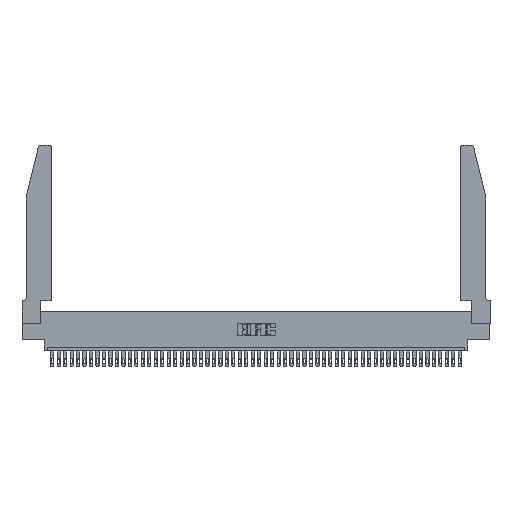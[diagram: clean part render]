
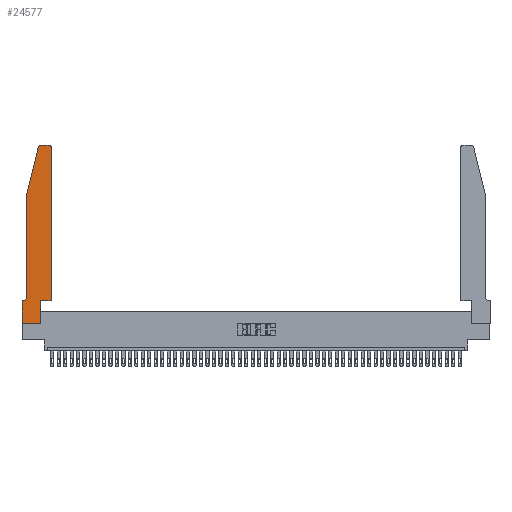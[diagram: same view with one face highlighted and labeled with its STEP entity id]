
A CAD part, top view. The second image highlights one B-rep face of the part: STEP entity #24577.
In plain terms, the highlighted planar face has unit normal (0, 0, 1).
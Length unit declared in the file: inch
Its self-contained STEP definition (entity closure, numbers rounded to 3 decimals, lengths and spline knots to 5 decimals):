
#942 = VERTEX_POINT ( 'NONE', #19809 ) ;
#1291 = VERTEX_POINT ( 'NONE', #23244 ) ;
#3203 = DIRECTION ( 'NONE',  ( 0., 1., 0. ) ) ;
#3223 = EDGE_CURVE ( 'NONE', #942, #12662, #13608, .T. ) ;
#3799 = CARTESIAN_POINT ( 'NONE',  ( 0., 0., 0.37 ) ) ;
#3910 = AXIS2_PLACEMENT_3D ( 'NONE', #31079, #4347, #4511 ) ;
#3929 = DIRECTION ( 'NONE',  ( 0., -1., 0. ) ) ;
#4347 = DIRECTION ( 'NONE',  ( 0., 0., -1. ) ) ;
#4511 = DIRECTION ( 'NONE',  ( -1., 0., 0. ) ) ;
#5018 = CARTESIAN_POINT ( 'NONE',  ( 0.4505, 0.35, 0.37 ) ) ;
#6240 = LINE ( 'NONE', #36328, #31482 ) ;
#6259 = ORIENTED_EDGE ( 'NONE', *, *, #28620, .T. ) ;
#6885 = VERTEX_POINT ( 'NONE', #7023 ) ;
#7023 = CARTESIAN_POINT ( 'NONE',  ( 0.0055, 0.35, 0.37 ) ) ;
#7160 = CARTESIAN_POINT ( 'NONE',  ( 0.2865, 0.35, 0.37 ) ) ;
#7862 = DIRECTION ( 'NONE',  ( 1., 0., 0. ) ) ;
#10143 = CARTESIAN_POINT ( 'NONE',  ( 0.2865, 0.35, 0.37 ) ) ;
#12261 = AXIS2_PLACEMENT_3D ( 'NONE', #22933, #26676, #34442 ) ;
#12622 = EDGE_CURVE ( 'NONE', #23413, #44478, #47587, .T. ) ;
#12662 = VERTEX_POINT ( 'NONE', #14508 ) ;
#13608 = CIRCLE ( 'NONE', #12261, 0.03 ) ;
#14015 = ORIENTED_EDGE ( 'NONE', *, *, #22513, .T. ) ;
#14288 = VERTEX_POINT ( 'NONE', #45154 ) ;
#14508 = CARTESIAN_POINT ( 'NONE',  ( 0.4205, 2.75, 0.37 ) ) ;
#14638 = EDGE_CURVE ( 'NONE', #30166, #6885, #20858, .T. ) ;
#15794 = CARTESIAN_POINT ( 'NONE',  ( 0.0755, 2., 0.37 ) ) ;
#15979 = EDGE_CURVE ( 'NONE', #1291, #19181, #23144, .T. ) ;
#16408 = LINE ( 'NONE', #47495, #32178 ) ;
#16878 = DIRECTION ( 'NONE',  ( -1., 0., 0. ) ) ;
#17016 = ORIENTED_EDGE ( 'NONE', *, *, #12622, .T. ) ;
#17214 = PLANE ( 'NONE',  #42375 ) ;
#17215 = ORIENTED_EDGE ( 'NONE', *, *, #38864, .T. ) ;
#18918 = VECTOR ( 'NONE', #7862, 39.37008 ) ;
#18948 = ORIENTED_EDGE ( 'NONE', *, *, #25670, .T. ) ;
#19085 = AXIS2_PLACEMENT_3D ( 'NONE', #39954, #24548, #27958 ) ;
#19181 = VERTEX_POINT ( 'NONE', #7160 ) ;
#19466 = LINE ( 'NONE', #3799, #18918 ) ;
#19809 = CARTESIAN_POINT ( 'NONE',  ( 0.4505, 2.72, 0.37 ) ) ;
#20485 = LINE ( 'NONE', #33072, #39870 ) ;
#20858 = CIRCLE ( 'NONE', #3910, 0.07 ) ;
#22232 = ORIENTED_EDGE ( 'NONE', *, *, #32112, .T. ) ;
#22513 = EDGE_CURVE ( 'NONE', #43325, #30166, #25351, .T. ) ;
#22933 = CARTESIAN_POINT ( 'NONE',  ( 0.4205, 2.72, 0.37 ) ) ;
#23144 = LINE ( 'NONE', #10143, #42506 ) ;
#23244 = CARTESIAN_POINT ( 'NONE',  ( 0.2865, 0., 0.37 ) ) ;
#23413 = VERTEX_POINT ( 'NONE', #28190 ) ;
#24548 = DIRECTION ( 'NONE',  ( 0., 0., 1. ) ) ;
#24577 = ADVANCED_FACE ( 'NONE', ( #46263 ), #17214, .T. ) ;
#25217 = LINE ( 'NONE', #38916, #40974 ) ;
#25351 = LINE ( 'NONE', #49342, #27148 ) ;
#25670 = EDGE_CURVE ( 'NONE', #12662, #23413, #38896, .T. ) ;
#26075 = CARTESIAN_POINT ( 'NONE',  ( 0.25487, 2.72718, 0.37 ) ) ;
#26676 = DIRECTION ( 'NONE',  ( 0., 0., 1. ) ) ;
#26905 = VECTOR ( 'NONE', #32027, 39.37008 ) ;
#27023 = DIRECTION ( 'NONE',  ( 0., -1., 0. ) ) ;
#27148 = VECTOR ( 'NONE', #27023, 39.37008 ) ;
#27455 = ORIENTED_EDGE ( 'NONE', *, *, #14638, .T. ) ;
#27585 = EDGE_CURVE ( 'NONE', #19181, #14288, #16408, .T. ) ;
#27894 = DIRECTION ( 'NONE',  ( 1., 0., 0. ) ) ;
#27958 = DIRECTION ( 'NONE',  ( 1., 0., 0. ) ) ;
#28190 = CARTESIAN_POINT ( 'NONE',  ( 0.284, 2.75, 0.37 ) ) ;
#28620 = EDGE_CURVE ( 'NONE', #14288, #942, #46807, .T. ) ;
#29042 = CARTESIAN_POINT ( 'NONE',  ( 0., 0.35, 0.37 ) ) ;
#30166 = VERTEX_POINT ( 'NONE', #39362 ) ;
#31028 = CARTESIAN_POINT ( 'NONE',  ( 0., 0., 0.37 ) ) ;
#31079 = CARTESIAN_POINT ( 'NONE',  ( 0.0055, 0.42, 0.37 ) ) ;
#31482 = VECTOR ( 'NONE', #16878, 39.37008 ) ;
#31575 = EDGE_LOOP ( 'NONE', ( #18948, #17016, #22232, #14015, #27455, #17215, #44981, #45176, #45067, #46803, #6259, #46067 ) ) ;
#32027 = DIRECTION ( 'NONE',  ( 0., 1., 0. ) ) ;
#32112 = EDGE_CURVE ( 'NONE', #44478, #43325, #20485, .T. ) ;
#32178 = VECTOR ( 'NONE', #27894, 39.37008 ) ;
#32766 = CARTESIAN_POINT ( 'NONE',  ( 0.2605, 2.75, 0.37 ) ) ;
#33072 = CARTESIAN_POINT ( 'NONE',  ( 0.0755, 2., 0.37 ) ) ;
#33648 = DIRECTION ( 'NONE',  ( -1., 0., 0. ) ) ;
#34442 = DIRECTION ( 'NONE',  ( 1., 0., 0. ) ) ;
#36328 = CARTESIAN_POINT ( 'NONE',  ( 0.0755, 0.35, 0.37 ) ) ;
#36683 = CARTESIAN_POINT ( 'NONE',  ( 0., 0.35, 0.37 ) ) ;
#38070 = VERTEX_POINT ( 'NONE', #31028 ) ;
#38864 = EDGE_CURVE ( 'NONE', #6885, #42929, #6240, .T. ) ;
#38896 = LINE ( 'NONE', #32766, #49169 ) ;
#38916 = CARTESIAN_POINT ( 'NONE',  ( 0., 0., 0.37 ) ) ;
#39362 = CARTESIAN_POINT ( 'NONE',  ( 0.0755, 0.42, 0.37 ) ) ;
#39870 = VECTOR ( 'NONE', #40896, 39.37008 ) ;
#39954 = CARTESIAN_POINT ( 'NONE',  ( 0.284, 2.72, 0.37 ) ) ;
#40572 = DIRECTION ( 'NONE',  ( 0., 0., 1. ) ) ;
#40896 = DIRECTION ( 'NONE',  ( -0.239, -0.971, 0. ) ) ;
#40966 = EDGE_CURVE ( 'NONE', #42929, #38070, #25217, .T. ) ;
#40974 = VECTOR ( 'NONE', #3929, 39.37008 ) ;
#42375 = AXIS2_PLACEMENT_3D ( 'NONE', #36683, #40572, #44451 ) ;
#42506 = VECTOR ( 'NONE', #3203, 39.37008 ) ;
#42929 = VERTEX_POINT ( 'NONE', #29042 ) ;
#43325 = VERTEX_POINT ( 'NONE', #15794 ) ;
#44451 = DIRECTION ( 'NONE',  ( 1., 0., 0. ) ) ;
#44478 = VERTEX_POINT ( 'NONE', #26075 ) ;
#44981 = ORIENTED_EDGE ( 'NONE', *, *, #40966, .T. ) ;
#45067 = ORIENTED_EDGE ( 'NONE', *, *, #15979, .T. ) ;
#45154 = CARTESIAN_POINT ( 'NONE',  ( 0.4505, 0.35, 0.37 ) ) ;
#45176 = ORIENTED_EDGE ( 'NONE', *, *, #49309, .T. ) ;
#46067 = ORIENTED_EDGE ( 'NONE', *, *, #3223, .T. ) ;
#46263 = FACE_OUTER_BOUND ( 'NONE', #31575, .T. ) ;
#46803 = ORIENTED_EDGE ( 'NONE', *, *, #27585, .T. ) ;
#46807 = LINE ( 'NONE', #5018, #26905 ) ;
#47495 = CARTESIAN_POINT ( 'NONE',  ( 0.4505, 0.35, 0.37 ) ) ;
#47587 = CIRCLE ( 'NONE', #19085, 0.03 ) ;
#49169 = VECTOR ( 'NONE', #33648, 39.37008 ) ;
#49309 = EDGE_CURVE ( 'NONE', #38070, #1291, #19466, .T. ) ;
#49342 = CARTESIAN_POINT ( 'NONE',  ( 0.0755, 2., 0.37 ) ) ;
